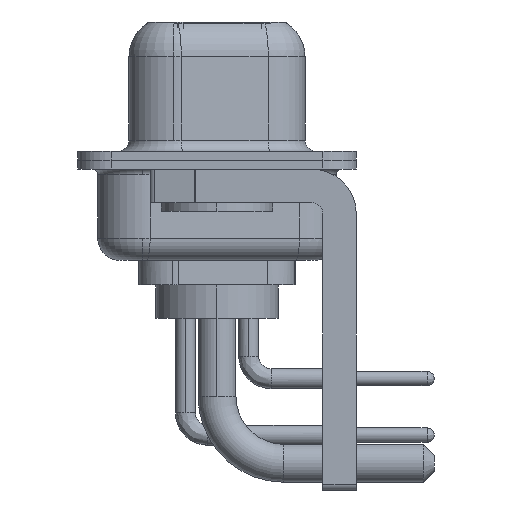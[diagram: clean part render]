
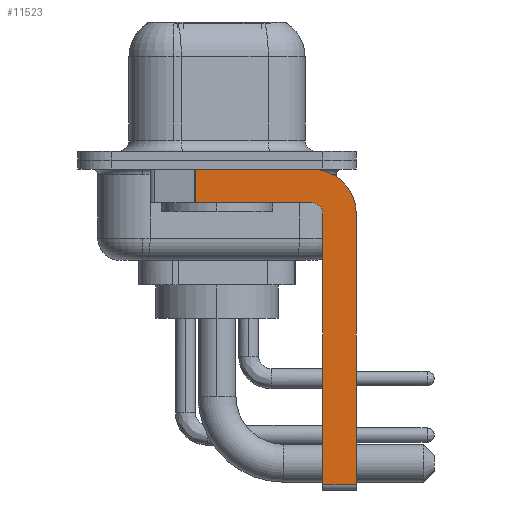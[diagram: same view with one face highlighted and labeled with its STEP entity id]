
A CAD part, left-side view. The second image highlights one B-rep face of the part: STEP entity #11523.
In plain terms, the highlighted planar face has unit normal (-1, 0, 0).
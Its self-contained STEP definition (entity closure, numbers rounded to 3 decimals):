
#678 = CARTESIAN_POINT ( 'NONE',  ( -2.9, -4.75, -2.4 ) ) ;
#821 = DIRECTION ( 'NONE',  ( 0., 0., 1. ) ) ;
#1267 = DIRECTION ( 'NONE',  ( 0., 0., -1. ) ) ;
#1821 = VERTEX_POINT ( 'NONE', #14004 ) ;
#1858 = DIRECTION ( 'NONE',  ( 0., 1., 0. ) ) ;
#2099 = DIRECTION ( 'NONE',  ( 0., -1., 0. ) ) ;
#2649 = CARTESIAN_POINT ( 'NONE',  ( -2.9, -6.25, -14.55 ) ) ;
#3356 = LINE ( 'NONE', #10932, #12417 ) ;
#3465 = EDGE_CURVE ( 'NONE', #19366, #5516, #9435, .T. ) ;
#3597 = ORIENTED_EDGE ( 'NONE', *, *, #3465, .F. ) ;
#3829 = CARTESIAN_POINT ( 'NONE',  ( -2.9, 0.978, -1.9 ) ) ;
#5363 = EDGE_CURVE ( 'NONE', #19366, #8661, #17358, .T. ) ;
#5516 = VERTEX_POINT ( 'NONE', #12277 ) ;
#5971 = VERTEX_POINT ( 'NONE', #16089 ) ;
#6056 = VERTEX_POINT ( 'NONE', #678 ) ;
#6068 = DIRECTION ( 'NONE',  ( 0., 0., -1. ) ) ;
#7268 = CARTESIAN_POINT ( 'NONE',  ( -2.9, -4.25, -2.4 ) ) ;
#7389 = DIRECTION ( 'NONE',  ( 0., 0., 1. ) ) ;
#7940 = CARTESIAN_POINT ( 'NONE',  ( -2.9, 3., -0.4 ) ) ;
#8661 = VERTEX_POINT ( 'NONE', #20147 ) ;
#8741 = EDGE_CURVE ( 'NONE', #21892, #13364, #3356, .T. ) ;
#8804 = EDGE_CURVE ( 'NONE', #1821, #8661, #19127, .T. ) ;
#8968 = CARTESIAN_POINT ( 'NONE',  ( -2.9, -4.25, -2.4 ) ) ;
#9435 = LINE ( 'NONE', #7940, #20689 ) ;
#9970 = CARTESIAN_POINT ( 'NONE',  ( -2.9, 0.978, -0.4 ) ) ;
#10261 = CARTESIAN_POINT ( 'NONE',  ( -2.9, -4.75, -14.8 ) ) ;
#10932 = CARTESIAN_POINT ( 'NONE',  ( -2.9, -6.25, -2.4 ) ) ;
#11085 = DIRECTION ( 'NONE',  ( 1., 0., 0. ) ) ;
#11301 = DIRECTION ( 'NONE',  ( 0., -1., 0. ) ) ;
#11418 = CARTESIAN_POINT ( 'NONE',  ( -2.9, -4.25, -1.9 ) ) ;
#11523 = ADVANCED_FACE ( 'NONE', ( #19038 ), #22800, .F. ) ;
#11608 = DIRECTION ( 'NONE',  ( -1., 0., 0. ) ) ;
#11967 = ORIENTED_EDGE ( 'NONE', *, *, #5363, .T. ) ;
#12277 = CARTESIAN_POINT ( 'NONE',  ( -2.9, -4.25, -0.4 ) ) ;
#12417 = VECTOR ( 'NONE', #14539, 1000. ) ;
#12943 = DIRECTION ( 'NONE',  ( 1., 0., 0. ) ) ;
#13364 = VERTEX_POINT ( 'NONE', #2649 ) ;
#13381 = ORIENTED_EDGE ( 'NONE', *, *, #18391, .F. ) ;
#13882 = CIRCLE ( 'NONE', #18646, 2. ) ;
#14004 = CARTESIAN_POINT ( 'NONE',  ( -2.9, -4.25, -1.9 ) ) ;
#14142 = ORIENTED_EDGE ( 'NONE', *, *, #8804, .F. ) ;
#14278 = EDGE_CURVE ( 'NONE', #5971, #13364, #17373, .T. ) ;
#14539 = DIRECTION ( 'NONE',  ( 0., 0., -1. ) ) ;
#14688 = EDGE_CURVE ( 'NONE', #6056, #1821, #20154, .T. ) ;
#15161 = VECTOR ( 'NONE', #1858, 1000. ) ;
#15423 = DIRECTION ( 'NONE',  ( 0., 0., -1. ) ) ;
#15509 = CARTESIAN_POINT ( 'NONE',  ( -2.9, -4.25, -14.55 ) ) ;
#16089 = CARTESIAN_POINT ( 'NONE',  ( -2.9, -4.75, -14.55 ) ) ;
#16540 = VECTOR ( 'NONE', #2099, 1000. ) ;
#17005 = ORIENTED_EDGE ( 'NONE', *, *, #23262, .F. ) ;
#17165 = CARTESIAN_POINT ( 'NONE',  ( -2.9, -4.25, -2.4 ) ) ;
#17249 = ORIENTED_EDGE ( 'NONE', *, *, #14688, .F. ) ;
#17358 = LINE ( 'NONE', #3829, #19548 ) ;
#17373 = LINE ( 'NONE', #15509, #16540 ) ;
#17499 = EDGE_LOOP ( 'NONE', ( #3597, #11967, #14142, #17249, #17005, #21402, #24149, #13381 ) ) ;
#18001 = AXIS2_PLACEMENT_3D ( 'NONE', #17165, #11085, #15423 ) ;
#18391 = EDGE_CURVE ( 'NONE', #5516, #21892, #13882, .T. ) ;
#18430 = VECTOR ( 'NONE', #821, 1000. ) ;
#18646 = AXIS2_PLACEMENT_3D ( 'NONE', #8968, #12943, #1267 ) ;
#19038 = FACE_OUTER_BOUND ( 'NONE', #17499, .T. ) ;
#19127 = LINE ( 'NONE', #11418, #15161 ) ;
#19366 = VERTEX_POINT ( 'NONE', #9970 ) ;
#19548 = VECTOR ( 'NONE', #6068, 1000. ) ;
#20147 = CARTESIAN_POINT ( 'NONE',  ( -2.9, 0.978, -1.9 ) ) ;
#20154 = CIRCLE ( 'NONE', #24519, 0.5 ) ;
#20689 = VECTOR ( 'NONE', #11301, 1000. ) ;
#21402 = ORIENTED_EDGE ( 'NONE', *, *, #14278, .T. ) ;
#21892 = VERTEX_POINT ( 'NONE', #23129 ) ;
#22800 = PLANE ( 'NONE',  #18001 ) ;
#23129 = CARTESIAN_POINT ( 'NONE',  ( -2.9, -6.25, -2.4 ) ) ;
#23262 = EDGE_CURVE ( 'NONE', #5971, #6056, #23353, .T. ) ;
#23353 = LINE ( 'NONE', #10261, #18430 ) ;
#24149 = ORIENTED_EDGE ( 'NONE', *, *, #8741, .F. ) ;
#24519 = AXIS2_PLACEMENT_3D ( 'NONE', #7268, #11608, #7389 ) ;
